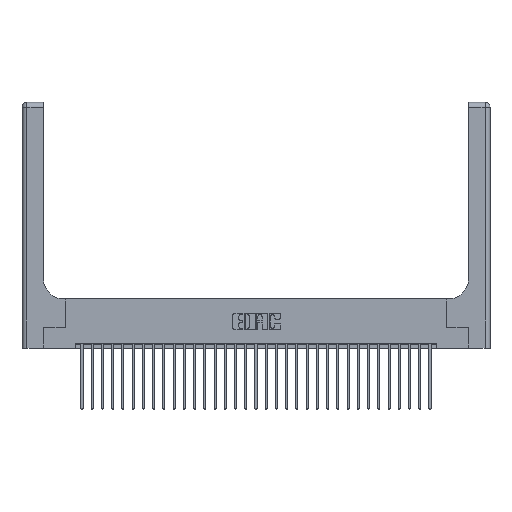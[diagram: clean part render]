
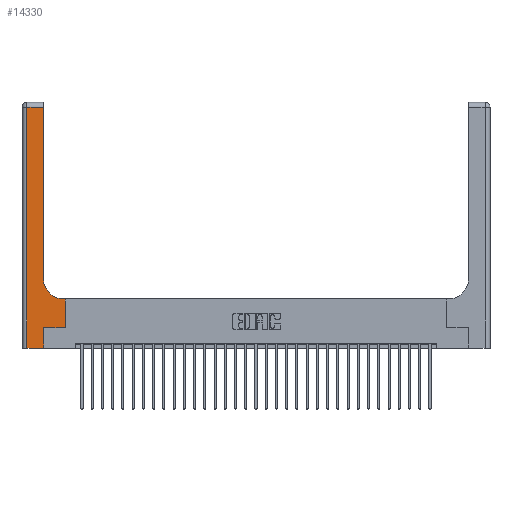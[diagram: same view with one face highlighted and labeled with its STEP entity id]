
A CAD part, top view. The second image highlights one B-rep face of the part: STEP entity #14330.
In plain terms, the highlighted planar face has unit normal (0, 0, 1).
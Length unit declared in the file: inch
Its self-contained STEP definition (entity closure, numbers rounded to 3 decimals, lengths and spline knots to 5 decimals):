
#969 = VERTEX_POINT ( 'NONE', #14510 ) ;
#1546 = DIRECTION ( 'NONE',  ( -1., 0., 0. ) ) ;
#3083 = DIRECTION ( 'NONE',  ( 1., 0., 0. ) ) ;
#3226 = VECTOR ( 'NONE', #1546, 39.37008 ) ;
#4168 = VERTEX_POINT ( 'NONE', #16304 ) ;
#4198 = EDGE_CURVE ( 'NONE', #20600, #4942, #27103, .T. ) ;
#4424 = CARTESIAN_POINT ( 'NONE',  ( 0.06, 2.94, 0.37 ) ) ;
#4872 = CARTESIAN_POINT ( 'NONE',  ( 0.528, 0.25, 0.37 ) ) ;
#4942 = VERTEX_POINT ( 'NONE', #17321 ) ;
#5336 = CARTESIAN_POINT ( 'NONE',  ( 0.528, 0.25, 0.37 ) ) ;
#5495 = CARTESIAN_POINT ( 'NONE',  ( 0., 0., 0.37 ) ) ;
#7207 = EDGE_CURVE ( 'NONE', #10262, #17111, #21290, .T. ) ;
#7300 = VECTOR ( 'NONE', #3083, 39.37008 ) ;
#7744 = DIRECTION ( 'NONE',  ( -1., 0., 0. ) ) ;
#7916 = LINE ( 'NONE', #15032, #18446 ) ;
#7964 = EDGE_CURVE ( 'NONE', #4942, #12699, #10417, .T. ) ;
#8252 = EDGE_CURVE ( 'NONE', #12699, #20075, #7916, .T. ) ;
#8639 = DIRECTION ( 'NONE',  ( 0., 1., 0. ) ) ;
#9352 = VECTOR ( 'NONE', #20462, 39.37008 ) ;
#9678 = EDGE_CURVE ( 'NONE', #20075, #10262, #22812, .T. ) ;
#10262 = VERTEX_POINT ( 'NONE', #4424 ) ;
#10417 = CIRCLE ( 'NONE', #16336, 0.25 ) ;
#11470 = CARTESIAN_POINT ( 'NONE',  ( 0., 2.94, 0.37 ) ) ;
#11526 = DIRECTION ( 'NONE',  ( 0., 0., -1. ) ) ;
#12699 = VERTEX_POINT ( 'NONE', #15502 ) ;
#12930 = LINE ( 'NONE', #5495, #7300 ) ;
#13221 = ORIENTED_EDGE ( 'NONE', *, *, #9678, .T. ) ;
#13801 = DIRECTION ( 'NONE',  ( 1., 0., 0. ) ) ;
#13897 = FACE_OUTER_BOUND ( 'NONE', #14992, .T. ) ;
#13964 = EDGE_CURVE ( 'NONE', #22398, #20600, #26497, .T. ) ;
#14330 = ADVANCED_FACE ( 'NONE', ( #13897 ), #26190, .F. ) ;
#14510 = CARTESIAN_POINT ( 'NONE',  ( 0.265, 0., 0.37 ) ) ;
#14992 = EDGE_LOOP ( 'NONE', ( #22655, #13221, #28095, #24780, #25252, #20656, #28670, #20859, #24206 ) ) ;
#15032 = CARTESIAN_POINT ( 'NONE',  ( 0.26, 3., 0.37 ) ) ;
#15252 = DIRECTION ( 'NONE',  ( -1., 0., 0. ) ) ;
#15502 = CARTESIAN_POINT ( 'NONE',  ( 0.26, 0.85, 0.37 ) ) ;
#16304 = CARTESIAN_POINT ( 'NONE',  ( 0.265, 0.25, 0.37 ) ) ;
#16336 = AXIS2_PLACEMENT_3D ( 'NONE', #24893, #11526, #13801 ) ;
#17024 = CARTESIAN_POINT ( 'NONE',  ( 0.26, 2.94, 0.37 ) ) ;
#17111 = VERTEX_POINT ( 'NONE', #26799 ) ;
#17160 = VECTOR ( 'NONE', #20230, 39.37008 ) ;
#17301 = CARTESIAN_POINT ( 'NONE',  ( 0., 3., 0.37 ) ) ;
#17321 = CARTESIAN_POINT ( 'NONE',  ( 0.51, 0.6, 0.37 ) ) ;
#17790 = CARTESIAN_POINT ( 'NONE',  ( 0.265, 0., 0.37 ) ) ;
#18446 = VECTOR ( 'NONE', #8639, 39.37008 ) ;
#18947 = CARTESIAN_POINT ( 'NONE',  ( 0.528, 0.6, 0.37 ) ) ;
#19555 = DIRECTION ( 'NONE',  ( 0., 0., -1. ) ) ;
#20075 = VERTEX_POINT ( 'NONE', #17024 ) ;
#20230 = DIRECTION ( 'NONE',  ( 0., 1., 0. ) ) ;
#20330 = DIRECTION ( 'NONE',  ( 0., -1., 0. ) ) ;
#20462 = DIRECTION ( 'NONE',  ( 0., 1., 0. ) ) ;
#20600 = VERTEX_POINT ( 'NONE', #18947 ) ;
#20656 = ORIENTED_EDGE ( 'NONE', *, *, #24718, .T. ) ;
#20859 = ORIENTED_EDGE ( 'NONE', *, *, #4198, .T. ) ;
#20872 = CARTESIAN_POINT ( 'NONE',  ( 0.26, 0.6, 0.37 ) ) ;
#20903 = DIRECTION ( 'NONE',  ( 1., 0., 0. ) ) ;
#21290 = LINE ( 'NONE', #22448, #24784 ) ;
#21655 = VECTOR ( 'NONE', #20903, 39.37008 ) ;
#21778 = AXIS2_PLACEMENT_3D ( 'NONE', #17301, #19555, #15252 ) ;
#22398 = VERTEX_POINT ( 'NONE', #5336 ) ;
#22448 = CARTESIAN_POINT ( 'NONE',  ( 0.06, 3., 0.37 ) ) ;
#22655 = ORIENTED_EDGE ( 'NONE', *, *, #8252, .T. ) ;
#22812 = LINE ( 'NONE', #11470, #3226 ) ;
#24206 = ORIENTED_EDGE ( 'NONE', *, *, #7964, .T. ) ;
#24551 = EDGE_CURVE ( 'NONE', #969, #4168, #26250, .T. ) ;
#24718 = EDGE_CURVE ( 'NONE', #4168, #22398, #27682, .T. ) ;
#24780 = ORIENTED_EDGE ( 'NONE', *, *, #24921, .T. ) ;
#24784 = VECTOR ( 'NONE', #20330, 39.37008 ) ;
#24893 = CARTESIAN_POINT ( 'NONE',  ( 0.51, 0.85, 0.37 ) ) ;
#24921 = EDGE_CURVE ( 'NONE', #17111, #969, #12930, .T. ) ;
#25002 = CARTESIAN_POINT ( 'NONE',  ( 0.265, 0.25, 0.37 ) ) ;
#25252 = ORIENTED_EDGE ( 'NONE', *, *, #24551, .T. ) ;
#26032 = VECTOR ( 'NONE', #7744, 39.37008 ) ;
#26190 = PLANE ( 'NONE',  #21778 ) ;
#26250 = LINE ( 'NONE', #17790, #17160 ) ;
#26497 = LINE ( 'NONE', #4872, #9352 ) ;
#26799 = CARTESIAN_POINT ( 'NONE',  ( 0.06, 0., 0.37 ) ) ;
#27103 = LINE ( 'NONE', #20872, #26032 ) ;
#27682 = LINE ( 'NONE', #25002, #21655 ) ;
#28095 = ORIENTED_EDGE ( 'NONE', *, *, #7207, .T. ) ;
#28670 = ORIENTED_EDGE ( 'NONE', *, *, #13964, .T. ) ;
